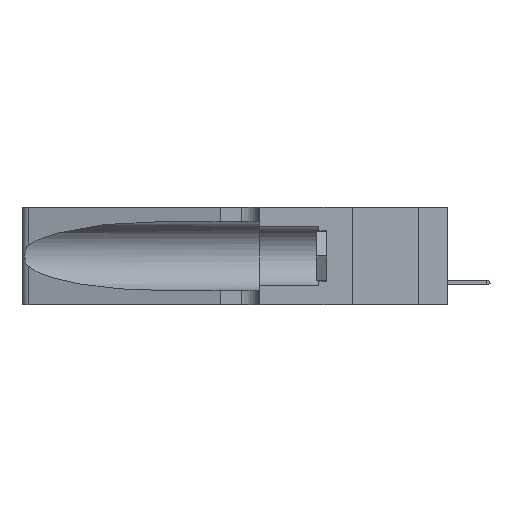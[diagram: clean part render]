
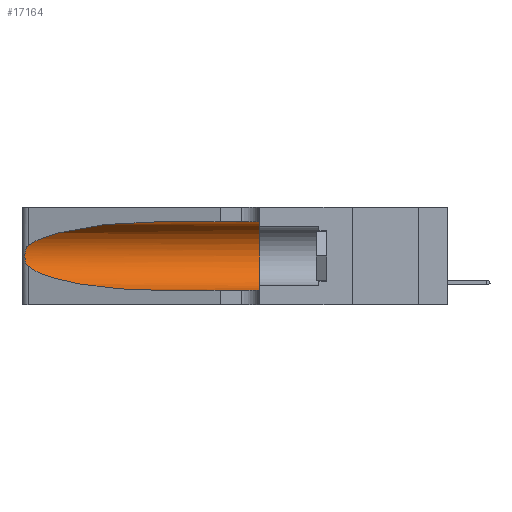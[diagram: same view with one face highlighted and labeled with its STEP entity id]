
A CAD part, left-side view. The second image highlights one B-rep face of the part: STEP entity #17164.
In plain terms, the highlighted cylindrical face has radius 3.308 mm (diameter 6.617 mm), a partial arc.
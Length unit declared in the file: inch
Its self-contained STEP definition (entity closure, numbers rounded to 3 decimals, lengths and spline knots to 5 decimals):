
#64 = DIRECTION ( 'NONE',  ( 0., 0., 1. ) ) ;
#1088 = VERTEX_POINT ( 'NONE', #18017 ) ;
#1278 = DIRECTION ( 'NONE',  ( 0., 0., -1. ) ) ;
#1417 = ORIENTED_EDGE ( 'NONE', *, *, #18913, .F. ) ;
#1666 = CARTESIAN_POINT ( 'NONE',  ( 0.1305, 0.72297, 0.05475 ) ) ;
#2137 = AXIS2_PLACEMENT_3D ( 'NONE', #6109, #15508, #64 ) ;
#2441 = CARTESIAN_POINT ( 'NONE',  ( 0.25789, 1.23486, 0.15765 ) ) ;
#2468 = VERTEX_POINT ( 'NONE', #11560 ) ;
#3100 = CARTESIAN_POINT ( 'NONE',  ( 0.1305, 0.35, 0.05475 ) ) ;
#3255 = CARTESIAN_POINT ( 'NONE',  ( 0.1305, 1.61858, 0.05475 ) ) ;
#3666 = CARTESIAN_POINT ( 'NONE',  ( 0.25787, 1.23484, 0.2124 ) ) ;
#3993 = CARTESIAN_POINT ( 'NONE',  ( 0.26018, 1.23835, 0.19895 ) ) ;
#4695 = CARTESIAN_POINT ( 'NONE',  ( 0.25487, 1.22718, 0.22369 ) ) ;
#4719 = CARTESIAN_POINT ( 'NONE',  ( 0.18966, 0.96281, 0.05475 ) ) ;
#5082 = EDGE_CURVE ( 'NONE', #1088, #2468, #12181, .T. ) ;
#5210 = ORIENTED_EDGE ( 'NONE', *, *, #6086, .T. ) ;
#5338 = ORIENTED_EDGE ( 'NONE', *, *, #5555, .F. ) ;
#5555 = EDGE_CURVE ( 'NONE', #6919, #9909, #16717, .T. ) ;
#5785 =( BOUNDED_CURVE ( )  B_SPLINE_CURVE ( 3, ( #15461, #18385, #4719, #1666 ),
 .UNSPECIFIED., .F., .F. ) 
 B_SPLINE_CURVE_WITH_KNOTS ( ( 4, 4 ),
 ( 3.44316, 4.71239 ),
 .UNSPECIFIED. ) 
 CURVE ( )  GEOMETRIC_REPRESENTATION_ITEM ( )  RATIONAL_B_SPLINE_CURVE ( ( 1., 0.87, 0.87, 1. ) ) 
 REPRESENTATION_ITEM ( '' )  );
#5792 = CARTESIAN_POINT ( 'NONE',  ( 0.25639, 1.23186, 0.15144 ) ) ;
#5883 = VECTOR ( 'NONE', #9502, 39.37008 ) ;
#6086 = EDGE_CURVE ( 'NONE', #2468, #11169, #5785, .T. ) ;
#6109 = CARTESIAN_POINT ( 'NONE',  ( 0.1305, 0.35, 0.185 ) ) ;
#6266 = CARTESIAN_POINT ( 'NONE',  ( 0.2373, 1.15595, 0.28018 ) ) ;
#6672 =( BOUNDED_CURVE ( )  B_SPLINE_CURVE ( 3, ( #7540, #16816, #6266, #7738 ),
 .UNSPECIFIED., .F., .T. ) 
 B_SPLINE_CURVE_WITH_KNOTS ( ( 4, 4 ),
 ( 1.5708, 2.84003 ),
 .UNSPECIFIED. ) 
 CURVE ( )  GEOMETRIC_REPRESENTATION_ITEM ( )  RATIONAL_B_SPLINE_CURVE ( ( 1., 0.87, 0.87, 1. ) ) 
 REPRESENTATION_ITEM ( '' )  );
#6897 = CARTESIAN_POINT ( 'NONE',  ( 0.26075, 1.23896, 0.178 ) ) ;
#6919 = VERTEX_POINT ( 'NONE', #11431 ) ;
#7540 = CARTESIAN_POINT ( 'NONE',  ( 0.1305, 0.72297, 0.31525 ) ) ;
#7738 = CARTESIAN_POINT ( 'NONE',  ( 0.25487, 1.22718, 0.22369 ) ) ;
#7772 = CARTESIAN_POINT ( 'NONE',  ( 0.25555, 1.22994, 0.2215 ) ) ;
#8581 = AXIS2_PLACEMENT_3D ( 'NONE', #19439, #10476, #1278 ) ;
#9090 = VECTOR ( 'NONE', #12489, 39.37008 ) ;
#9104 = CARTESIAN_POINT ( 'NONE',  ( 0.1305, 1.61858, 0.31525 ) ) ;
#9163 = EDGE_LOOP ( 'NONE', ( #11641, #10417, #5210, #10710, #5338, #1417 ) ) ;
#9502 = DIRECTION ( 'NONE',  ( 0., -1., 0. ) ) ;
#9647 = CARTESIAN_POINT ( 'NONE',  ( 0.25639, 1.23184, 0.21858 ) ) ;
#9909 = VERTEX_POINT ( 'NONE', #3100 ) ;
#10417 = ORIENTED_EDGE ( 'NONE', *, *, #5082, .T. ) ;
#10476 = DIRECTION ( 'NONE',  ( 0., -1., 0. ) ) ;
#10482 = CARTESIAN_POINT ( 'NONE',  ( 0.25487, 1.22718, 0.14631 ) ) ;
#10621 = CYLINDRICAL_SURFACE ( 'NONE', #8581, 0.13025 ) ;
#10710 = ORIENTED_EDGE ( 'NONE', *, *, #14422, .T. ) ;
#11169 = VERTEX_POINT ( 'NONE', #14043 ) ;
#11431 = CARTESIAN_POINT ( 'NONE',  ( 0.1305, 0.35, 0.31525 ) ) ;
#11556 = CARTESIAN_POINT ( 'NONE',  ( 0.26075, 1.23896, 0.19203 ) ) ;
#11560 = CARTESIAN_POINT ( 'NONE',  ( 0.25487, 1.22718, 0.14631 ) ) ;
#11641 = ORIENTED_EDGE ( 'NONE', *, *, #17178, .T. ) ;
#12181 = B_SPLINE_CURVE_WITH_KNOTS ( 'NONE', 3,
 ( #4695, #7772, #9647, #3666, #14344, #3993, #11556, #6897, #13074, #17690, #2441, #5792, #16551, #10482 ),
 .UNSPECIFIED., .F., .F.,
 ( 4, 2, 2, 2, 2, 2, 4 ),
 ( 0., 0.00027, 0.00053, 0.00107, 0.0016, 0.00187, 0.00214 ),
 .UNSPECIFIED. ) ;
#12323 = LINE ( 'NONE', #3255, #5883 ) ;
#12489 = DIRECTION ( 'NONE',  ( 0., -1., 0. ) ) ;
#13074 = CARTESIAN_POINT ( 'NONE',  ( 0.26017, 1.23833, 0.17102 ) ) ;
#13171 = VERTEX_POINT ( 'NONE', #13682 ) ;
#13682 = CARTESIAN_POINT ( 'NONE',  ( 0.1305, 0.72297, 0.31525 ) ) ;
#13925 = FACE_OUTER_BOUND ( 'NONE', #9163, .T. ) ;
#14043 = CARTESIAN_POINT ( 'NONE',  ( 0.1305, 0.72297, 0.05475 ) ) ;
#14077 = LINE ( 'NONE', #9104, #9090 ) ;
#14344 = CARTESIAN_POINT ( 'NONE',  ( 0.25854, 1.2359, 0.20912 ) ) ;
#14422 = EDGE_CURVE ( 'NONE', #11169, #9909, #12323, .T. ) ;
#15461 = CARTESIAN_POINT ( 'NONE',  ( 0.25487, 1.22718, 0.14631 ) ) ;
#15508 = DIRECTION ( 'NONE',  ( 0., 1., 0. ) ) ;
#16551 = CARTESIAN_POINT ( 'NONE',  ( 0.25555, 1.22993, 0.14849 ) ) ;
#16717 = CIRCLE ( 'NONE', #2137, 0.13025 ) ;
#16816 = CARTESIAN_POINT ( 'NONE',  ( 0.18966, 0.96281, 0.31525 ) ) ;
#17164 = ADVANCED_FACE ( 'NONE', ( #13925 ), #10621, .F. ) ;
#17178 = EDGE_CURVE ( 'NONE', #13171, #1088, #6672, .T. ) ;
#17690 = CARTESIAN_POINT ( 'NONE',  ( 0.25856, 1.23593, 0.16098 ) ) ;
#18017 = CARTESIAN_POINT ( 'NONE',  ( 0.25487, 1.22718, 0.22369 ) ) ;
#18385 = CARTESIAN_POINT ( 'NONE',  ( 0.2373, 1.15595, 0.08982 ) ) ;
#18913 = EDGE_CURVE ( 'NONE', #13171, #6919, #14077, .T. ) ;
#19439 = CARTESIAN_POINT ( 'NONE',  ( 0.1305, 1.61858, 0.185 ) ) ;
